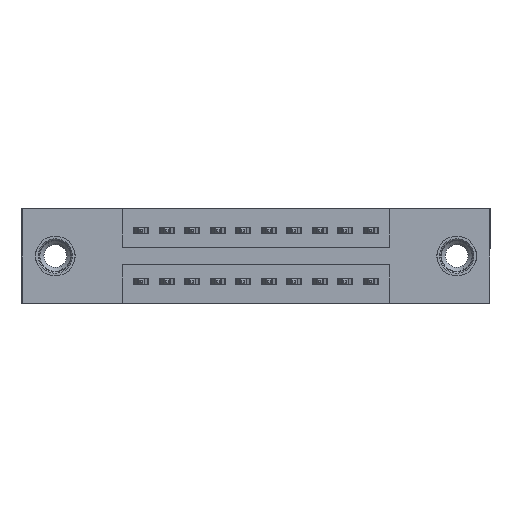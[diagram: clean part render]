
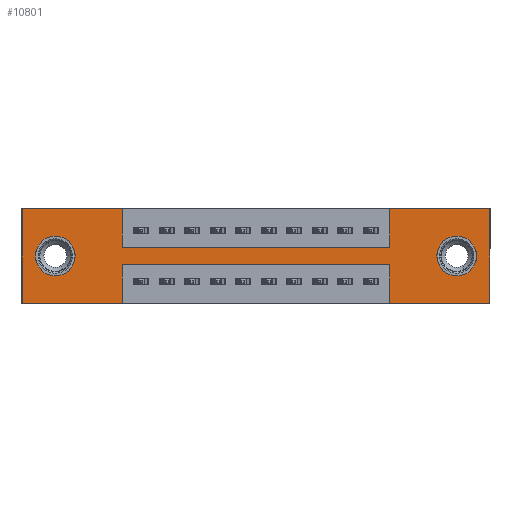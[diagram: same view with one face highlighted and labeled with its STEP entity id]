
A CAD part, front view. The second image highlights one B-rep face of the part: STEP entity #10801.
In plain terms, the highlighted planar face has unit normal (0, -1, 0).
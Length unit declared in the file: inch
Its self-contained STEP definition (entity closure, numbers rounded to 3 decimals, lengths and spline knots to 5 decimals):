
#139 = EDGE_CURVE ( 'NONE', #8749, #3415, #9519, .T. ) ;
#315 = FACE_BOUND ( 'NONE', #7344, .T. ) ;
#671 = CARTESIAN_POINT ( 'NONE',  ( 0.13, 0., -0.185 ) ) ;
#731 = AXIS2_PLACEMENT_3D ( 'NONE', #3552, #11281, #4659 ) ;
#856 = VERTEX_POINT ( 'NONE', #7447 ) ;
#896 = VECTOR ( 'NONE', #7939, 39.37008 ) ;
#1159 = ORIENTED_EDGE ( 'NONE', *, *, #11976, .F. ) ;
#1239 = ORIENTED_EDGE ( 'NONE', *, *, #139, .F. ) ;
#1399 = VECTOR ( 'NONE', #6312, 39.37008 ) ;
#1446 = DIRECTION ( 'NONE',  ( 0., 0., -1. ) ) ;
#1463 = CARTESIAN_POINT ( 'NONE',  ( 1.4425, 0., 0. ) ) ;
#1480 = CARTESIAN_POINT ( 'NONE',  ( 0.3925, 0., 0. ) ) ;
#1563 = AXIS2_PLACEMENT_3D ( 'NONE', #11235, #4613, #12337 ) ;
#1798 = CARTESIAN_POINT ( 'NONE',  ( 1.835, 0., 0. ) ) ;
#1817 = DIRECTION ( 'NONE',  ( 0., 0., 1. ) ) ;
#1851 = LINE ( 'NONE', #1463, #12097 ) ;
#2071 = CARTESIAN_POINT ( 'NONE',  ( 1.4425, 0., -0.37 ) ) ;
#2075 = EDGE_CURVE ( 'NONE', #8522, #8749, #10723, .T. ) ;
#2186 = CARTESIAN_POINT ( 'NONE',  ( 1.835, 0., 0. ) ) ;
#2227 = VECTOR ( 'NONE', #1446, 39.37008 ) ;
#2319 = CIRCLE ( 'NONE', #3474, 0.078 ) ;
#2452 = ORIENTED_EDGE ( 'NONE', *, *, #2075, .F. ) ;
#2782 = ORIENTED_EDGE ( 'NONE', *, *, #8861, .F. ) ;
#3017 = DIRECTION ( 'NONE',  ( -1., 0., 0. ) ) ;
#3173 = CARTESIAN_POINT ( 'NONE',  ( 1.4425, 0., 0. ) ) ;
#3208 = ORIENTED_EDGE ( 'NONE', *, *, #8839, .F. ) ;
#3210 = DIRECTION ( 'NONE',  ( 0., -1., 0. ) ) ;
#3300 = ORIENTED_EDGE ( 'NONE', *, *, #11828, .F. ) ;
#3328 = CARTESIAN_POINT ( 'NONE',  ( 0., 0., 0. ) ) ;
#3340 = ORIENTED_EDGE ( 'NONE', *, *, #9428, .F. ) ;
#3368 = AXIS2_PLACEMENT_3D ( 'NONE', #671, #8419, #1817 ) ;
#3377 = ORIENTED_EDGE ( 'NONE', *, *, #8779, .T. ) ;
#3415 = VERTEX_POINT ( 'NONE', #4235 ) ;
#3474 = AXIS2_PLACEMENT_3D ( 'NONE', #5656, #13384, #6744 ) ;
#3502 = ORIENTED_EDGE ( 'NONE', *, *, #13169, .F. ) ;
#3552 = CARTESIAN_POINT ( 'NONE',  ( 0.13, 0., -0.185 ) ) ;
#4204 = VERTEX_POINT ( 'NONE', #2186 ) ;
#4235 = CARTESIAN_POINT ( 'NONE',  ( 1.4425, 0., -0.15 ) ) ;
#4248 = LINE ( 'NONE', #4992, #10099 ) ;
#4532 = LINE ( 'NONE', #7075, #10044 ) ;
#4613 = DIRECTION ( 'NONE',  ( 0., 1., 0. ) ) ;
#4659 = DIRECTION ( 'NONE',  ( 0., 0., 1. ) ) ;
#4670 = DIRECTION ( 'NONE',  ( -1., 0., 0. ) ) ;
#4992 = CARTESIAN_POINT ( 'NONE',  ( 1.4425, 0., -0.37 ) ) ;
#5208 = CARTESIAN_POINT ( 'NONE',  ( 0., 0., 0. ) ) ;
#5373 = VECTOR ( 'NONE', #8278, 39.37008 ) ;
#5423 = VERTEX_POINT ( 'NONE', #10000 ) ;
#5586 = VERTEX_POINT ( 'NONE', #8025 ) ;
#5614 = ORIENTED_EDGE ( 'NONE', *, *, #10997, .T. ) ;
#5626 = ORIENTED_EDGE ( 'NONE', *, *, #7532, .T. ) ;
#5656 = CARTESIAN_POINT ( 'NONE',  ( 1.705, 0., -0.185 ) ) ;
#5742 = CARTESIAN_POINT ( 'NONE',  ( 0., 0., -0.37 ) ) ;
#6034 = EDGE_CURVE ( 'NONE', #856, #8522, #13503, .T. ) ;
#6227 = EDGE_LOOP ( 'NONE', ( #10117, #5614 ) ) ;
#6311 = VECTOR ( 'NONE', #10683, 39.37008 ) ;
#6312 = DIRECTION ( 'NONE',  ( 0., 0., 1. ) ) ;
#6325 = CARTESIAN_POINT ( 'NONE',  ( 0.3925, 0., 0. ) ) ;
#6624 = LINE ( 'NONE', #1798, #6311 ) ;
#6736 = CARTESIAN_POINT ( 'NONE',  ( 0.3925, 0., -0.22 ) ) ;
#6744 = DIRECTION ( 'NONE',  ( 0., 0., -1. ) ) ;
#6885 = VERTEX_POINT ( 'NONE', #8971 ) ;
#7029 = CARTESIAN_POINT ( 'NONE',  ( 0., 0., -0.37 ) ) ;
#7052 = VERTEX_POINT ( 'NONE', #7029 ) ;
#7075 = CARTESIAN_POINT ( 'NONE',  ( 0.3925, 0., -0.22 ) ) ;
#7109 = EDGE_CURVE ( 'NONE', #12414, #11078, #11294, .T. ) ;
#7192 = EDGE_CURVE ( 'NONE', #10699, #11425, #13158, .T. ) ;
#7319 = CARTESIAN_POINT ( 'NONE',  ( 0.3925, 0., -0.15 ) ) ;
#7344 = EDGE_LOOP ( 'NONE', ( #3377, #5626 ) ) ;
#7366 = CARTESIAN_POINT ( 'NONE',  ( 0., 0., -0.37 ) ) ;
#7447 = CARTESIAN_POINT ( 'NONE',  ( 0., 0., 0. ) ) ;
#7532 = EDGE_CURVE ( 'NONE', #7611, #6885, #8980, .T. ) ;
#7611 = VERTEX_POINT ( 'NONE', #13501 ) ;
#7686 = AXIS2_PLACEMENT_3D ( 'NONE', #8661, #3210, #10937 ) ;
#7702 = EDGE_LOOP ( 'NONE', ( #11899, #3300, #13441, #1159, #3340, #2782, #3502, #1239, #2452, #7806, #13071, #3208 ) ) ;
#7753 = CARTESIAN_POINT ( 'NONE',  ( 0.3925, 0., -0.15 ) ) ;
#7806 = ORIENTED_EDGE ( 'NONE', *, *, #6034, .F. ) ;
#7866 = DIRECTION ( 'NONE',  ( 1., 0., 0. ) ) ;
#7939 = DIRECTION ( 'NONE',  ( 1., 0., 0. ) ) ;
#8025 = CARTESIAN_POINT ( 'NONE',  ( 1.4425, 0., -0.22 ) ) ;
#8067 = DIRECTION ( 'NONE',  ( 0., 0., 1. ) ) ;
#8278 = DIRECTION ( 'NONE',  ( 0., 0., -1. ) ) ;
#8419 = DIRECTION ( 'NONE',  ( 0., 1., 0. ) ) ;
#8522 = VERTEX_POINT ( 'NONE', #6325 ) ;
#8600 = CARTESIAN_POINT ( 'NONE',  ( 0.13, 0., -0.263 ) ) ;
#8661 = CARTESIAN_POINT ( 'NONE',  ( 0., 0., -0.37 ) ) ;
#8749 = VERTEX_POINT ( 'NONE', #7753 ) ;
#8779 = EDGE_CURVE ( 'NONE', #6885, #7611, #2319, .T. ) ;
#8839 = EDGE_CURVE ( 'NONE', #11078, #7052, #10111, .T. ) ;
#8861 = EDGE_CURVE ( 'NONE', #10271, #4204, #9763, .T. ) ;
#8971 = CARTESIAN_POINT ( 'NONE',  ( 1.705, 0., -0.107 ) ) ;
#8980 = CIRCLE ( 'NONE', #1563, 0.078 ) ;
#9075 = CARTESIAN_POINT ( 'NONE',  ( 0., 0., 0. ) ) ;
#9110 = CARTESIAN_POINT ( 'NONE',  ( 0.3925, 0., -0.37 ) ) ;
#9424 = CARTESIAN_POINT ( 'NONE',  ( 0.3925, 0., -0.37 ) ) ;
#9428 = EDGE_CURVE ( 'NONE', #4204, #5423, #6624, .T. ) ;
#9519 = LINE ( 'NONE', #7319, #12133 ) ;
#9763 = LINE ( 'NONE', #9075, #896 ) ;
#9816 = PLANE ( 'NONE',  #7686 ) ;
#10000 = CARTESIAN_POINT ( 'NONE',  ( 1.835, 0., -0.37 ) ) ;
#10031 = EDGE_CURVE ( 'NONE', #10806, #5586, #4248, .T. ) ;
#10044 = VECTOR ( 'NONE', #10482, 39.37008 ) ;
#10099 = VECTOR ( 'NONE', #12680, 39.37008 ) ;
#10111 = LINE ( 'NONE', #5742, #12701 ) ;
#10117 = ORIENTED_EDGE ( 'NONE', *, *, #7192, .T. ) ;
#10255 = LINE ( 'NONE', #5208, #1399 ) ;
#10271 = VERTEX_POINT ( 'NONE', #3173 ) ;
#10482 = DIRECTION ( 'NONE',  ( -1., 0., 0. ) ) ;
#10606 = VECTOR ( 'NONE', #13990, 39.37008 ) ;
#10683 = DIRECTION ( 'NONE',  ( 0., 0., -1. ) ) ;
#10699 = VERTEX_POINT ( 'NONE', #10746 ) ;
#10713 = EDGE_CURVE ( 'NONE', #7052, #856, #10255, .T. ) ;
#10723 = LINE ( 'NONE', #1480, #2227 ) ;
#10746 = CARTESIAN_POINT ( 'NONE',  ( 0.13, 0., -0.107 ) ) ;
#10801 = ADVANCED_FACE ( 'NONE', ( #315, #11832, #11488 ), #9816, .T. ) ;
#10806 = VERTEX_POINT ( 'NONE', #2071 ) ;
#10918 = VECTOR ( 'NONE', #3017, 39.37008 ) ;
#10937 = DIRECTION ( 'NONE',  ( 0., 0., -1. ) ) ;
#10997 = EDGE_CURVE ( 'NONE', #11425, #10699, #11986, .T. ) ;
#11078 = VERTEX_POINT ( 'NONE', #9110 ) ;
#11235 = CARTESIAN_POINT ( 'NONE',  ( 1.705, 0., -0.185 ) ) ;
#11281 = DIRECTION ( 'NONE',  ( 0., 1., 0. ) ) ;
#11294 = LINE ( 'NONE', #9424, #5373 ) ;
#11425 = VERTEX_POINT ( 'NONE', #8600 ) ;
#11488 = FACE_OUTER_BOUND ( 'NONE', #7702, .T. ) ;
#11828 = EDGE_CURVE ( 'NONE', #5586, #12414, #4532, .T. ) ;
#11832 = FACE_BOUND ( 'NONE', #6227, .T. ) ;
#11899 = ORIENTED_EDGE ( 'NONE', *, *, #7109, .F. ) ;
#11976 = EDGE_CURVE ( 'NONE', #5423, #10806, #13793, .T. ) ;
#11986 = CIRCLE ( 'NONE', #731, 0.078 ) ;
#12097 = VECTOR ( 'NONE', #8067, 39.37008 ) ;
#12133 = VECTOR ( 'NONE', #7866, 39.37008 ) ;
#12337 = DIRECTION ( 'NONE',  ( 0., 0., -1. ) ) ;
#12414 = VERTEX_POINT ( 'NONE', #6736 ) ;
#12680 = DIRECTION ( 'NONE',  ( 0., 0., 1. ) ) ;
#12701 = VECTOR ( 'NONE', #4670, 39.37008 ) ;
#13071 = ORIENTED_EDGE ( 'NONE', *, *, #10713, .F. ) ;
#13158 = CIRCLE ( 'NONE', #3368, 0.078 ) ;
#13169 = EDGE_CURVE ( 'NONE', #3415, #10271, #1851, .T. ) ;
#13384 = DIRECTION ( 'NONE',  ( 0., 1., 0. ) ) ;
#13441 = ORIENTED_EDGE ( 'NONE', *, *, #10031, .F. ) ;
#13501 = CARTESIAN_POINT ( 'NONE',  ( 1.705, 0., -0.263 ) ) ;
#13503 = LINE ( 'NONE', #3328, #10606 ) ;
#13793 = LINE ( 'NONE', #7366, #10918 ) ;
#13990 = DIRECTION ( 'NONE',  ( 1., 0., 0. ) ) ;
